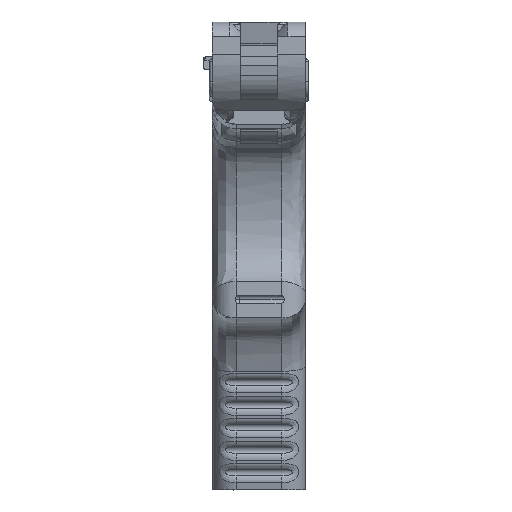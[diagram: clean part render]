
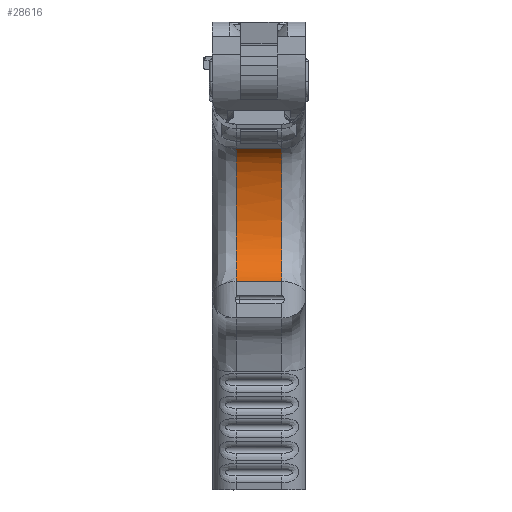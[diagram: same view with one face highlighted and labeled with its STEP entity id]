
A CAD part, front view. The second image highlights one B-rep face of the part: STEP entity #28616.
In plain terms, the highlighted free-form (B-spline) face has degree [5, 1] with [20, 2] control points.
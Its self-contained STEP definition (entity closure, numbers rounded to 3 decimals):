
#2283=B_SPLINE_CURVE_WITH_KNOTS('',3,(#57529,#57530,#57531,#57532,#57533,
#57534,#57535,#57536,#57537,#57538,#57539,#57540),.UNSPECIFIED.,.F.,.F.,
(4,1,1,1,1,1,1,1,1,4),(0.,0.484,0.968,
1.452,1.936,2.177,2.419,2.903,
3.145,3.387),.UNSPECIFIED.);
#2286=B_SPLINE_CURVE_WITH_KNOTS('',3,(#57774,#57775,#57776,#57777,#57778,
#57779,#57780,#57781,#57782,#57783,#57784,#57785),.UNSPECIFIED.,.F.,.F.,
(4,1,1,1,1,1,1,1,1,4),(0.,0.242,0.363,0.484,
0.968,1.452,1.936,2.419,2.903,
3.387),.UNSPECIFIED.);
#3029=B_SPLINE_SURFACE_WITH_KNOTS('',5,1,((#57732,#57733),(#57734,#57735),
(#57736,#57737),(#57738,#57739),(#57740,#57741),(#57742,#57743),(#57744,
#57745),(#57746,#57747),(#57748,#57749),(#57750,#57751),(#57752,#57753),
(#57754,#57755),(#57756,#57757),(#57758,#57759),(#57760,#57761),(#57762,
#57763),(#57764,#57765),(#57766,#57767),(#57768,#57769),(#57770,#57771)),
 .UNSPECIFIED.,.F.,.F.,.F.,(6,1,1,1,1,1,1,1,1,1,1,1,1,1,1,6),(2,2),(-1.,
-0.96,-0.92,-0.88,-0.84,-0.8,-0.76,-0.72,-0.68,-0.64,-0.6,-0.56,-0.52,-0.48,
-0.44,-0.423),(0.,15.6),.UNSPECIFIED.);
#4292=FACE_OUTER_BOUND('',#5921,.T.);
#5921=EDGE_LOOP('',(#25598,#25599,#25600,#25601));
#7919=LINE('',#57238,#10180);
#7963=LINE('',#57773,#10224);
#10180=VECTOR('',#33877,10.);
#10224=VECTOR('',#34011,10.);
#12172=VERTEX_POINT('',#42120);
#13680=VERTEX_POINT('',#56636);
#13751=VERTEX_POINT('',#57514);
#13753=VERTEX_POINT('',#57772);
#17773=EDGE_CURVE('',#12172,#13680,#7919,.T.);
#17834=EDGE_CURVE('',#13751,#12172,#2283,.T.);
#17839=EDGE_CURVE('',#13751,#13753,#7963,.T.);
#17840=EDGE_CURVE('',#13680,#13753,#2286,.T.);
#25598=ORIENTED_EDGE('',*,*,#17834,.F.);
#25599=ORIENTED_EDGE('',*,*,#17839,.T.);
#25600=ORIENTED_EDGE('',*,*,#17840,.F.);
#25601=ORIENTED_EDGE('',*,*,#17773,.F.);
#28616=ADVANCED_FACE('',(#4292),#3029,.F.);
#33877=DIRECTION('',(1.,0.,0.));
#34011=DIRECTION('',(1.,0.,0.));
#42120=CARTESIAN_POINT('',(-3.991,-33.833,59.383));
#56636=CARTESIAN_POINT('',(3.709,-33.833,59.383));
#57238=CARTESIAN_POINT('',(0.,-33.833,59.383));
#57514=CARTESIAN_POINT('',(-3.991,-33.833,37.));
#57529=CARTESIAN_POINT('Ctrl Pts',(-3.991,-33.833,
37.));
#57530=CARTESIAN_POINT('Ctrl Pts',(-3.991,-32.807,
37.559));
#57531=CARTESIAN_POINT('Ctrl Pts',(-3.991,-31.061,
38.956));
#57532=CARTESIAN_POINT('Ctrl Pts',(-3.991,-29.426,
41.874));
#57533=CARTESIAN_POINT('Ctrl Pts',(-3.991,-28.795,
45.545));
#57534=CARTESIAN_POINT('Ctrl Pts',(-3.991,-29.034,
48.964));
#57535=CARTESIAN_POINT('Ctrl Pts',(-3.991,-29.568,
51.742));
#57536=CARTESIAN_POINT('Ctrl Pts',(-3.991,-30.306,
54.481));
#57537=CARTESIAN_POINT('Ctrl Pts',(-3.991,-31.322,
56.884));
#57538=CARTESIAN_POINT('Ctrl Pts',(-3.991,-32.6,
58.471));
#57539=CARTESIAN_POINT('Ctrl Pts',(-3.991,-33.385,
59.1));
#57540=CARTESIAN_POINT('Ctrl Pts',(-3.991,-33.833,
59.383));
#57732=CARTESIAN_POINT('Ctrl Pts',(-65.,-33.833,37.));
#57733=CARTESIAN_POINT('Ctrl Pts',(91.,-33.833,37.));
#57734=CARTESIAN_POINT('Ctrl Pts',(-65.,-33.535,37.162));
#57735=CARTESIAN_POINT('Ctrl Pts',(91.,-33.535,37.162));
#57736=CARTESIAN_POINT('Ctrl Pts',(-65.,-32.961,37.506));
#57737=CARTESIAN_POINT('Ctrl Pts',(91.,-32.961,37.506));
#57738=CARTESIAN_POINT('Ctrl Pts',(-65.,-32.168,38.078));
#57739=CARTESIAN_POINT('Ctrl Pts',(91.,-32.168,38.078));
#57740=CARTESIAN_POINT('Ctrl Pts',(-65.,-31.245,38.956));
#57741=CARTESIAN_POINT('Ctrl Pts',(91.,-31.245,38.956));
#57742=CARTESIAN_POINT('Ctrl Pts',(-65.,-30.319,40.243));
#57743=CARTESIAN_POINT('Ctrl Pts',(91.,-30.319,40.243));
#57744=CARTESIAN_POINT('Ctrl Pts',(-65.,-29.621,41.718));
#57745=CARTESIAN_POINT('Ctrl Pts',(91.,-29.621,41.718));
#57746=CARTESIAN_POINT('Ctrl Pts',(-65.,-29.153,43.372));
#57747=CARTESIAN_POINT('Ctrl Pts',(91.,-29.153,43.372));
#57748=CARTESIAN_POINT('Ctrl Pts',(-65.,-28.915,45.19));
#57749=CARTESIAN_POINT('Ctrl Pts',(91.,-28.915,45.19));
#57750=CARTESIAN_POINT('Ctrl Pts',(-65.,-28.897,47.141));
#57751=CARTESIAN_POINT('Ctrl Pts',(91.,-28.897,47.141));
#57752=CARTESIAN_POINT('Ctrl Pts',(-65.,-29.084,49.178));
#57753=CARTESIAN_POINT('Ctrl Pts',(91.,-29.084,49.178));
#57754=CARTESIAN_POINT('Ctrl Pts',(-65.,-29.444,51.23));
#57755=CARTESIAN_POINT('Ctrl Pts',(91.,-29.444,51.23));
#57756=CARTESIAN_POINT('Ctrl Pts',(-65.,-29.937,53.208));
#57757=CARTESIAN_POINT('Ctrl Pts',(91.,-29.937,53.208));
#57758=CARTESIAN_POINT('Ctrl Pts',(-65.,-30.537,55.026));
#57759=CARTESIAN_POINT('Ctrl Pts',(91.,-30.537,55.026));
#57760=CARTESIAN_POINT('Ctrl Pts',(-65.,-31.24,56.616));
#57761=CARTESIAN_POINT('Ctrl Pts',(91.,-31.24,56.616));
#57762=CARTESIAN_POINT('Ctrl Pts',(-65.,-31.991,57.795));
#57763=CARTESIAN_POINT('Ctrl Pts',(91.,-31.991,57.795));
#57764=CARTESIAN_POINT('Ctrl Pts',(-65.,-32.711,58.563));
#57765=CARTESIAN_POINT('Ctrl Pts',(91.,-32.711,58.563));
#57766=CARTESIAN_POINT('Ctrl Pts',(-65.,-33.317,59.044));
#57767=CARTESIAN_POINT('Ctrl Pts',(91.,-33.317,59.044));
#57768=CARTESIAN_POINT('Ctrl Pts',(-65.,-33.712,59.306));
#57769=CARTESIAN_POINT('Ctrl Pts',(91.,-33.712,59.306));
#57770=CARTESIAN_POINT('Ctrl Pts',(-65.,-33.833,59.383));
#57771=CARTESIAN_POINT('Ctrl Pts',(91.,-33.833,59.383));
#57772=CARTESIAN_POINT('',(3.709,-33.833,37.));
#57773=CARTESIAN_POINT('',(0.,-33.833,37.));
#57774=CARTESIAN_POINT('Ctrl Pts',(3.709,-33.833,59.383));
#57775=CARTESIAN_POINT('Ctrl Pts',(3.709,-33.385,59.1));
#57776=CARTESIAN_POINT('Ctrl Pts',(3.709,-32.796,58.634));
#57777=CARTESIAN_POINT('Ctrl Pts',(3.709,-32.121,57.876));
#57778=CARTESIAN_POINT('Ctrl Pts',(3.709,-31.195,56.591));
#57779=CARTESIAN_POINT('Ctrl Pts',(3.709,-30.052,53.861));
#57780=CARTESIAN_POINT('Ctrl Pts',(3.709,-29.082,49.633));
#57781=CARTESIAN_POINT('Ctrl Pts',(3.709,-28.794,45.549));
#57782=CARTESIAN_POINT('Ctrl Pts',(3.709,-29.426,41.87));
#57783=CARTESIAN_POINT('Ctrl Pts',(3.709,-31.061,38.956));
#57784=CARTESIAN_POINT('Ctrl Pts',(3.709,-32.807,37.559));
#57785=CARTESIAN_POINT('Ctrl Pts',(3.709,-33.833,37.));
